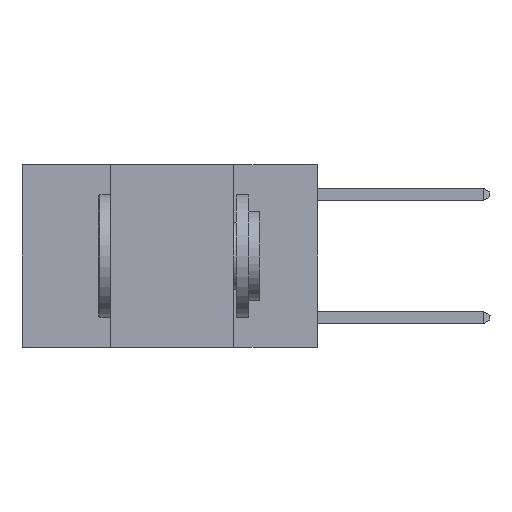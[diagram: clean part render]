
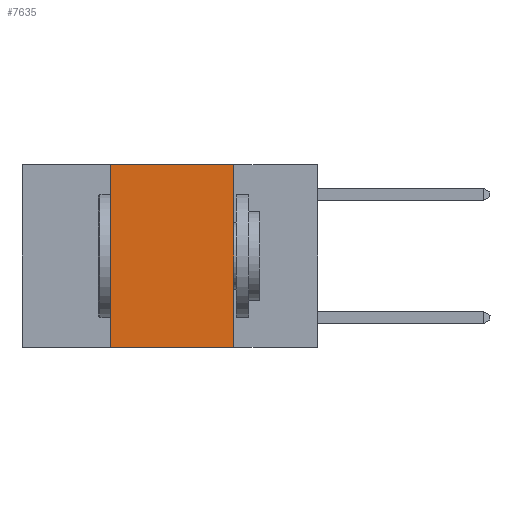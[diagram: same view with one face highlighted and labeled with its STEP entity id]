
A CAD part, left-side view. The second image highlights one B-rep face of the part: STEP entity #7635.
In plain terms, the highlighted planar face has unit normal (-1, 0, 0).
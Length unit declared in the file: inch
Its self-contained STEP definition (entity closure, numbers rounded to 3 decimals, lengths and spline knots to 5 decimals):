
#59 = EDGE_CURVE ( 'NONE', #11971, #10473, #13565, .T. ) ;
#68 = CARTESIAN_POINT ( 'NONE',  ( 0., 0.17, 0. ) ) ;
#490 = DIRECTION ( 'NONE',  ( 0., 0., 1. ) ) ;
#2154 = CARTESIAN_POINT ( 'NONE',  ( 0., 0.17, 0. ) ) ;
#2235 = LINE ( 'NONE', #4879, #12560 ) ;
#3376 = LINE ( 'NONE', #13942, #13156 ) ;
#3672 = ORIENTED_EDGE ( 'NONE', *, *, #17781, .F. ) ;
#4429 = FACE_OUTER_BOUND ( 'NONE', #9491, .T. ) ;
#4879 = CARTESIAN_POINT ( 'NONE',  ( 0., 0.6, -0.37 ) ) ;
#6314 = DIRECTION ( 'NONE',  ( 0., -1., 0. ) ) ;
#6936 = VERTEX_POINT ( 'NONE', #16289 ) ;
#7106 = DIRECTION ( 'NONE',  ( 1., 0., 0. ) ) ;
#7191 = PLANE ( 'NONE',  #13678 ) ;
#7288 = DIRECTION ( 'NONE',  ( 0., 0., -1. ) ) ;
#7635 = ADVANCED_FACE ( 'NONE', ( #4429 ), #7191, .F. ) ;
#7929 = DIRECTION ( 'NONE',  ( 0., -1., 0. ) ) ;
#9491 = EDGE_LOOP ( 'NONE', ( #18424, #16479, #3672, #17755 ) ) ;
#10061 = CARTESIAN_POINT ( 'NONE',  ( 0., 0.6, 0. ) ) ;
#10473 = VERTEX_POINT ( 'NONE', #68 ) ;
#10901 = LINE ( 'NONE', #2154, #10948 ) ;
#10948 = VECTOR ( 'NONE', #16596, 39.37008 ) ;
#11454 = VERTEX_POINT ( 'NONE', #12590 ) ;
#11971 = VERTEX_POINT ( 'NONE', #13207 ) ;
#12044 = VECTOR ( 'NONE', #7929, 39.37008 ) ;
#12560 = VECTOR ( 'NONE', #6314, 39.37008 ) ;
#12590 = CARTESIAN_POINT ( 'NONE',  ( 0., 0.42, -0.37 ) ) ;
#13156 = VECTOR ( 'NONE', #490, 39.37008 ) ;
#13207 = CARTESIAN_POINT ( 'NONE',  ( 0., 0.42, 0. ) ) ;
#13521 = EDGE_CURVE ( 'NONE', #10473, #6936, #10901, .T. ) ;
#13565 = LINE ( 'NONE', #15147, #12044 ) ;
#13678 = AXIS2_PLACEMENT_3D ( 'NONE', #10061, #7106, #7288 ) ;
#13942 = CARTESIAN_POINT ( 'NONE',  ( 0., 0.42, 0. ) ) ;
#15147 = CARTESIAN_POINT ( 'NONE',  ( 0., 0.6, 0. ) ) ;
#16289 = CARTESIAN_POINT ( 'NONE',  ( 0., 0.17, -0.37 ) ) ;
#16407 = EDGE_CURVE ( 'NONE', #11454, #6936, #2235, .T. ) ;
#16479 = ORIENTED_EDGE ( 'NONE', *, *, #59, .F. ) ;
#16596 = DIRECTION ( 'NONE',  ( 0., 0., -1. ) ) ;
#17755 = ORIENTED_EDGE ( 'NONE', *, *, #16407, .T. ) ;
#17781 = EDGE_CURVE ( 'NONE', #11454, #11971, #3376, .T. ) ;
#18424 = ORIENTED_EDGE ( 'NONE', *, *, #13521, .F. ) ;
